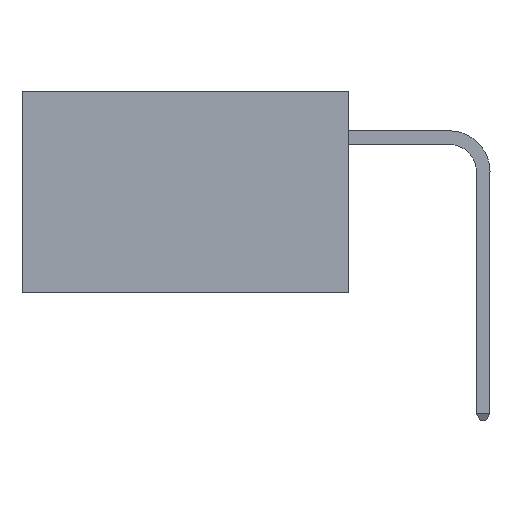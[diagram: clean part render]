
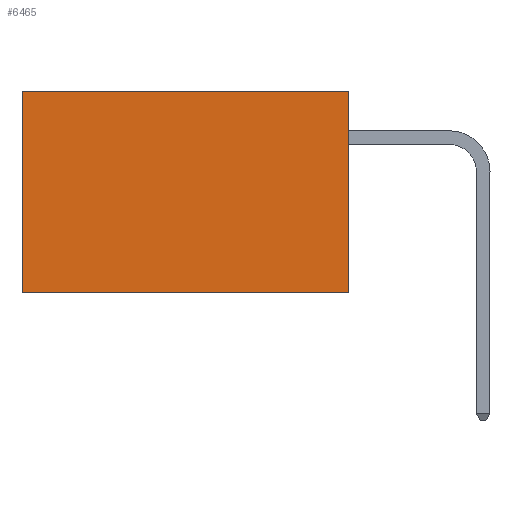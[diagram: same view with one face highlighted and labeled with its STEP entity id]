
A CAD part, left-side view. The second image highlights one B-rep face of the part: STEP entity #6465.
In plain terms, the highlighted planar face has unit normal (-1, 0, 0).
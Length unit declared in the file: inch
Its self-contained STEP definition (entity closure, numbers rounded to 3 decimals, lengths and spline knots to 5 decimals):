
#87 = EDGE_CURVE ( 'NONE', #6600, #1828, #3324, .T. ) ;
#124 = CARTESIAN_POINT ( 'NONE',  ( 0.2875, 0., -0.37 ) ) ;
#145 = CARTESIAN_POINT ( 'NONE',  ( 0.2875, 0.6, 0. ) ) ;
#474 = EDGE_CURVE ( 'NONE', #2442, #6600, #6847, .T. ) ;
#597 = DIRECTION ( 'NONE',  ( 0., 1., 0. ) ) ;
#1086 = DIRECTION ( 'NONE',  ( 0., 0., -1. ) ) ;
#1673 = DIRECTION ( 'NONE',  ( 1., 0., 0. ) ) ;
#1828 = VERTEX_POINT ( 'NONE', #4770 ) ;
#2442 = VERTEX_POINT ( 'NONE', #3932 ) ;
#2583 = EDGE_CURVE ( 'NONE', #5883, #1828, #7921, .T. ) ;
#2783 = VECTOR ( 'NONE', #8634, 39.37008 ) ;
#2838 = LINE ( 'NONE', #8645, #2783 ) ;
#2866 = CARTESIAN_POINT ( 'NONE',  ( 0.2875, 0.6, 0. ) ) ;
#3179 = CARTESIAN_POINT ( 'NONE',  ( 0.2875, 0., -0.37 ) ) ;
#3324 = LINE ( 'NONE', #2866, #3491 ) ;
#3491 = VECTOR ( 'NONE', #1086, 39.37008 ) ;
#3535 = AXIS2_PLACEMENT_3D ( 'NONE', #6105, #1673, #6709 ) ;
#3932 = CARTESIAN_POINT ( 'NONE',  ( 0.2875, 0., 0. ) ) ;
#4534 = ORIENTED_EDGE ( 'NONE', *, *, #5770, .F. ) ;
#4687 = ORIENTED_EDGE ( 'NONE', *, *, #2583, .F. ) ;
#4770 = CARTESIAN_POINT ( 'NONE',  ( 0.2875, 0.6, -0.37 ) ) ;
#5770 = EDGE_CURVE ( 'NONE', #2442, #5883, #2838, .T. ) ;
#5883 = VERTEX_POINT ( 'NONE', #3179 ) ;
#6083 = PLANE ( 'NONE',  #3535 ) ;
#6105 = CARTESIAN_POINT ( 'NONE',  ( 0.2875, 0., 0. ) ) ;
#6465 = ADVANCED_FACE ( 'NONE', ( #7418 ), #6083, .F. ) ;
#6600 = VERTEX_POINT ( 'NONE', #145 ) ;
#6688 = VECTOR ( 'NONE', #8807, 39.37008 ) ;
#6709 = DIRECTION ( 'NONE',  ( 0., 0., -1. ) ) ;
#6847 = LINE ( 'NONE', #8256, #6688 ) ;
#7159 = VECTOR ( 'NONE', #597, 39.37008 ) ;
#7406 = EDGE_LOOP ( 'NONE', ( #8333, #4687, #4534, #7954 ) ) ;
#7418 = FACE_OUTER_BOUND ( 'NONE', #7406, .T. ) ;
#7921 = LINE ( 'NONE', #124, #7159 ) ;
#7954 = ORIENTED_EDGE ( 'NONE', *, *, #474, .T. ) ;
#8256 = CARTESIAN_POINT ( 'NONE',  ( 0.2875, 0., 0. ) ) ;
#8333 = ORIENTED_EDGE ( 'NONE', *, *, #87, .T. ) ;
#8634 = DIRECTION ( 'NONE',  ( 0., 0., -1. ) ) ;
#8645 = CARTESIAN_POINT ( 'NONE',  ( 0.2875, 0., 0. ) ) ;
#8807 = DIRECTION ( 'NONE',  ( 0., 1., 0. ) ) ;
